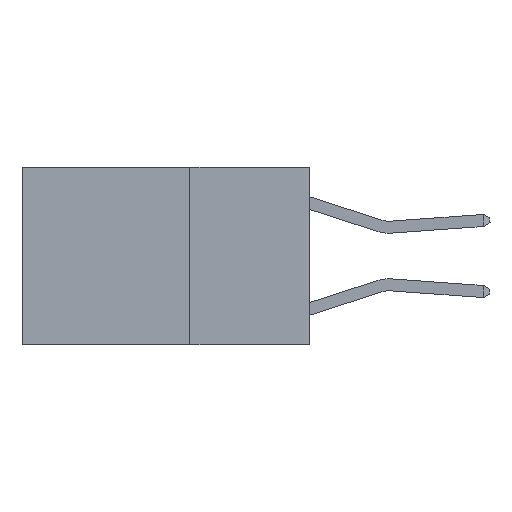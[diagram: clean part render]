
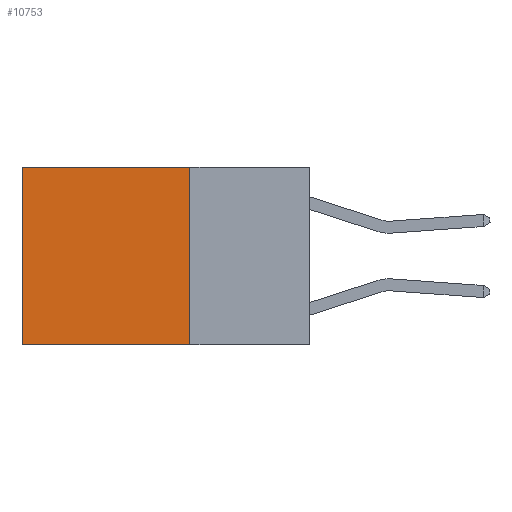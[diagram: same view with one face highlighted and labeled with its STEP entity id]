
A CAD part, left-side view. The second image highlights one B-rep face of the part: STEP entity #10753.
In plain terms, the highlighted planar face has unit normal (-1, 0, 0).
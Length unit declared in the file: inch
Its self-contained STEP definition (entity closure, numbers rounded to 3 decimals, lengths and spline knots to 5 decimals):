
#15 = LINE ( 'NONE', #583, #9593 ) ;
#115 = EDGE_LOOP ( 'NONE', ( #5257, #8708, #8367, #3235 ) ) ;
#460 = VERTEX_POINT ( 'NONE', #1671 ) ;
#505 = CARTESIAN_POINT ( 'NONE',  ( 0.2625, 0.25, 0. ) ) ;
#583 = CARTESIAN_POINT ( 'NONE',  ( 0.2625, 0.25, 0. ) ) ;
#743 = EDGE_CURVE ( 'NONE', #4984, #460, #10257, .T. ) ;
#1040 = EDGE_CURVE ( 'NONE', #6800, #5350, #15, .T. ) ;
#1671 = CARTESIAN_POINT ( 'NONE',  ( 0.2625, 0.6, -0.37 ) ) ;
#2481 = CARTESIAN_POINT ( 'NONE',  ( 0.2625, 0.25, 0. ) ) ;
#2782 = EDGE_CURVE ( 'NONE', #6800, #4984, #9469, .T. ) ;
#3205 = VECTOR ( 'NONE', #5647, 39.37008 ) ;
#3235 = ORIENTED_EDGE ( 'NONE', *, *, #2782, .T. ) ;
#3299 = CARTESIAN_POINT ( 'NONE',  ( 0.2625, 0.6, 0. ) ) ;
#4169 = DIRECTION ( 'NONE',  ( 0., 1., 0. ) ) ;
#4312 = DIRECTION ( 'NONE',  ( 0., 1., 0. ) ) ;
#4571 = CARTESIAN_POINT ( 'NONE',  ( 0.2625, 0.25, 0. ) ) ;
#4984 = VERTEX_POINT ( 'NONE', #3299 ) ;
#5257 = ORIENTED_EDGE ( 'NONE', *, *, #743, .T. ) ;
#5350 = VERTEX_POINT ( 'NONE', #9162 ) ;
#5519 = DIRECTION ( 'NONE',  ( 1., 0., 0. ) ) ;
#5647 = DIRECTION ( 'NONE',  ( 0., 0., -1. ) ) ;
#6086 = CARTESIAN_POINT ( 'NONE',  ( 0.2625, 0.25, -0.37 ) ) ;
#6109 = DIRECTION ( 'NONE',  ( 0., 0., -1. ) ) ;
#6800 = VERTEX_POINT ( 'NONE', #2481 ) ;
#7398 = EDGE_CURVE ( 'NONE', #5350, #460, #8156, .T. ) ;
#7716 = FACE_OUTER_BOUND ( 'NONE', #115, .T. ) ;
#7898 = VECTOR ( 'NONE', #4312, 39.37008 ) ;
#8156 = LINE ( 'NONE', #6086, #7898 ) ;
#8367 = ORIENTED_EDGE ( 'NONE', *, *, #1040, .F. ) ;
#8708 = ORIENTED_EDGE ( 'NONE', *, *, #7398, .F. ) ;
#8973 = PLANE ( 'NONE',  #11109 ) ;
#9162 = CARTESIAN_POINT ( 'NONE',  ( 0.2625, 0.25, -0.37 ) ) ;
#9469 = LINE ( 'NONE', #505, #9741 ) ;
#9593 = VECTOR ( 'NONE', #6109, 39.37008 ) ;
#9741 = VECTOR ( 'NONE', #4169, 39.37008 ) ;
#9961 = CARTESIAN_POINT ( 'NONE',  ( 0.2625, 0.6, 0. ) ) ;
#10257 = LINE ( 'NONE', #9961, #3205 ) ;
#10753 = ADVANCED_FACE ( 'NONE', ( #7716 ), #8973, .F. ) ;
#11109 = AXIS2_PLACEMENT_3D ( 'NONE', #4571, #5519, #11437 ) ;
#11437 = DIRECTION ( 'NONE',  ( 0., 0., -1. ) ) ;
